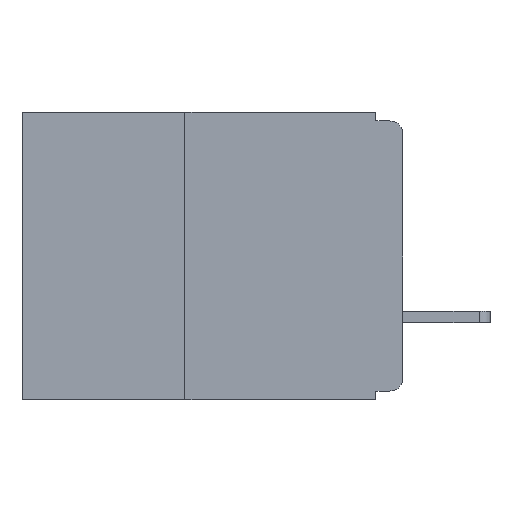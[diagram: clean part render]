
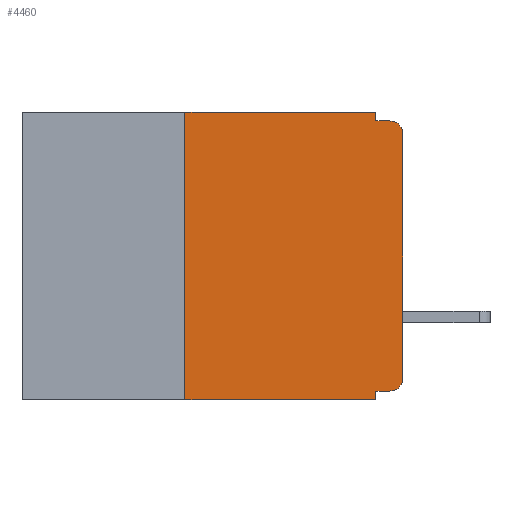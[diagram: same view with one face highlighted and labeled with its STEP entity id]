
A CAD part, left-side view. The second image highlights one B-rep face of the part: STEP entity #4460.
In plain terms, the highlighted planar face has unit normal (-1, 0, 0).
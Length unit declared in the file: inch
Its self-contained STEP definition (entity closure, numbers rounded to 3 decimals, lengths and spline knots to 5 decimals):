
#86 = EDGE_CURVE ( 'NONE', #28460, #4605, #3990, .T. ) ;
#453 = ORIENTED_EDGE ( 'NONE', *, *, #33506, .T. ) ;
#1036 = VECTOR ( 'NONE', #4978, 39.37008 ) ;
#1941 = DIRECTION ( 'NONE',  ( -1., 0., 0. ) ) ;
#2078 = CARTESIAN_POINT ( 'NONE',  ( 0., 0.031, -0.32 ) ) ;
#2536 = VECTOR ( 'NONE', #11048, 39.37008 ) ;
#2762 = CARTESIAN_POINT ( 'NONE',  ( 0., 0., -0.01 ) ) ;
#3634 = DIRECTION ( 'NONE',  ( 0., -1., 0. ) ) ;
#3878 = CARTESIAN_POINT ( 'NONE',  ( 0., 0.031, 0. ) ) ;
#3990 = LINE ( 'NONE', #3878, #18574 ) ;
#4026 = EDGE_CURVE ( 'NONE', #14923, #10702, #20819, .T. ) ;
#4460 = ADVANCED_FACE ( 'NONE', ( #19936 ), #7016, .F. ) ;
#4605 = VERTEX_POINT ( 'NONE', #21261 ) ;
#4807 = ORIENTED_EDGE ( 'NONE', *, *, #7833, .F. ) ;
#4946 = LINE ( 'NONE', #21172, #25756 ) ;
#4978 = DIRECTION ( 'NONE',  ( 0., -1., 0. ) ) ;
#5294 = DIRECTION ( 'NONE',  ( 0., 1., 0. ) ) ;
#6363 = AXIS2_PLACEMENT_3D ( 'NONE', #30639, #12516, #31214 ) ;
#7016 = PLANE ( 'NONE',  #6363 ) ;
#7833 = EDGE_CURVE ( 'NONE', #4605, #10702, #9872, .T. ) ;
#8545 = DIRECTION ( 'NONE',  ( 0., 0., -1. ) ) ;
#9872 = LINE ( 'NONE', #2762, #2536 ) ;
#10043 = CARTESIAN_POINT ( 'NONE',  ( 0., 0.031, -0.33 ) ) ;
#10154 = EDGE_CURVE ( 'NONE', #20671, #32046, #12435, .T. ) ;
#10268 = DIRECTION ( 'NONE',  ( -1., 0., 0. ) ) ;
#10417 = CARTESIAN_POINT ( 'NONE',  ( 0., 0.031, -0.33 ) ) ;
#10702 = VERTEX_POINT ( 'NONE', #14465 ) ;
#11029 = LINE ( 'NONE', #20075, #19190 ) ;
#11048 = DIRECTION ( 'NONE',  ( 0., -1., 0. ) ) ;
#11998 = DIRECTION ( 'NONE',  ( 0., 0., 1. ) ) ;
#12435 = LINE ( 'NONE', #20269, #25955 ) ;
#12516 = DIRECTION ( 'NONE',  ( 1., 0., 0. ) ) ;
#14465 = CARTESIAN_POINT ( 'NONE',  ( 0., 0.015, -0.01 ) ) ;
#14923 = VERTEX_POINT ( 'NONE', #23010 ) ;
#15909 = VERTEX_POINT ( 'NONE', #16317 ) ;
#16218 = VECTOR ( 'NONE', #5294, 39.37008 ) ;
#16317 = CARTESIAN_POINT ( 'NONE',  ( 0., 0.015, -0.32 ) ) ;
#16389 = ORIENTED_EDGE ( 'NONE', *, *, #18151, .T. ) ;
#17005 = ORIENTED_EDGE ( 'NONE', *, *, #10154, .F. ) ;
#17563 = VERTEX_POINT ( 'NONE', #10417 ) ;
#17717 = VERTEX_POINT ( 'NONE', #19157 ) ;
#18151 = EDGE_CURVE ( 'NONE', #15909, #17717, #32704, .T. ) ;
#18158 = EDGE_CURVE ( 'NONE', #17717, #14923, #4946, .T. ) ;
#18416 = CARTESIAN_POINT ( 'NONE',  ( 0., 0.015, -0.025 ) ) ;
#18574 = VECTOR ( 'NONE', #8545, 39.37008 ) ;
#18603 = EDGE_LOOP ( 'NONE', ( #30926, #27932, #4807, #26254, #25774, #17005, #453, #20177, #22841, #16389 ) ) ;
#19157 = CARTESIAN_POINT ( 'NONE',  ( 0., 0., -0.305 ) ) ;
#19190 = VECTOR ( 'NONE', #3634, 39.37008 ) ;
#19894 = LINE ( 'NONE', #10043, #33864 ) ;
#19935 = EDGE_CURVE ( 'NONE', #21190, #17563, #19894, .T. ) ;
#19936 = FACE_OUTER_BOUND ( 'NONE', #18603, .T. ) ;
#20075 = CARTESIAN_POINT ( 'NONE',  ( 0., 0.437, -0.33 ) ) ;
#20177 = ORIENTED_EDGE ( 'NONE', *, *, #19935, .F. ) ;
#20269 = CARTESIAN_POINT ( 'NONE',  ( 0., 0.25, -0.33 ) ) ;
#20671 = VERTEX_POINT ( 'NONE', #32204 ) ;
#20819 = CIRCLE ( 'NONE', #22379, 0.015 ) ;
#21172 = CARTESIAN_POINT ( 'NONE',  ( 0., 0., 0. ) ) ;
#21175 = DIRECTION ( 'NONE',  ( 0., 0., -1. ) ) ;
#21190 = VERTEX_POINT ( 'NONE', #2078 ) ;
#21261 = CARTESIAN_POINT ( 'NONE',  ( 0., 0.031, -0.01 ) ) ;
#22379 = AXIS2_PLACEMENT_3D ( 'NONE', #18416, #1941, #21175 ) ;
#22385 = AXIS2_PLACEMENT_3D ( 'NONE', #26448, #10268, #29071 ) ;
#22841 = ORIENTED_EDGE ( 'NONE', *, *, #26414, .F. ) ;
#23010 = CARTESIAN_POINT ( 'NONE',  ( 0., 0., -0.025 ) ) ;
#23730 = LINE ( 'NONE', #29185, #1036 ) ;
#24338 = CARTESIAN_POINT ( 'NONE',  ( 0., 0., -0.32 ) ) ;
#25756 = VECTOR ( 'NONE', #28960, 39.37008 ) ;
#25774 = ORIENTED_EDGE ( 'NONE', *, *, #27453, .F. ) ;
#25955 = VECTOR ( 'NONE', #11998, 39.37008 ) ;
#26254 = ORIENTED_EDGE ( 'NONE', *, *, #86, .F. ) ;
#26414 = EDGE_CURVE ( 'NONE', #15909, #21190, #31175, .T. ) ;
#26448 = CARTESIAN_POINT ( 'NONE',  ( 0., 0.015, -0.305 ) ) ;
#27453 = EDGE_CURVE ( 'NONE', #32046, #28460, #23730, .T. ) ;
#27932 = ORIENTED_EDGE ( 'NONE', *, *, #4026, .T. ) ;
#28460 = VERTEX_POINT ( 'NONE', #30697 ) ;
#28960 = DIRECTION ( 'NONE',  ( 0., 0., 1. ) ) ;
#29027 = CARTESIAN_POINT ( 'NONE',  ( 0., 0.25, 0. ) ) ;
#29071 = DIRECTION ( 'NONE',  ( 0., 0., -1. ) ) ;
#29185 = CARTESIAN_POINT ( 'NONE',  ( 0., 0.437, 0. ) ) ;
#30639 = CARTESIAN_POINT ( 'NONE',  ( 0., 0.437, 0. ) ) ;
#30697 = CARTESIAN_POINT ( 'NONE',  ( 0., 0.031, 0. ) ) ;
#30926 = ORIENTED_EDGE ( 'NONE', *, *, #18158, .T. ) ;
#31175 = LINE ( 'NONE', #24338, #16218 ) ;
#31214 = DIRECTION ( 'NONE',  ( 0., 0., -1. ) ) ;
#31474 = DIRECTION ( 'NONE',  ( 0., 0., -1. ) ) ;
#32046 = VERTEX_POINT ( 'NONE', #29027 ) ;
#32204 = CARTESIAN_POINT ( 'NONE',  ( 0., 0.25, -0.33 ) ) ;
#32704 = CIRCLE ( 'NONE', #22385, 0.015 ) ;
#33506 = EDGE_CURVE ( 'NONE', #20671, #17563, #11029, .T. ) ;
#33864 = VECTOR ( 'NONE', #31474, 39.37008 ) ;
